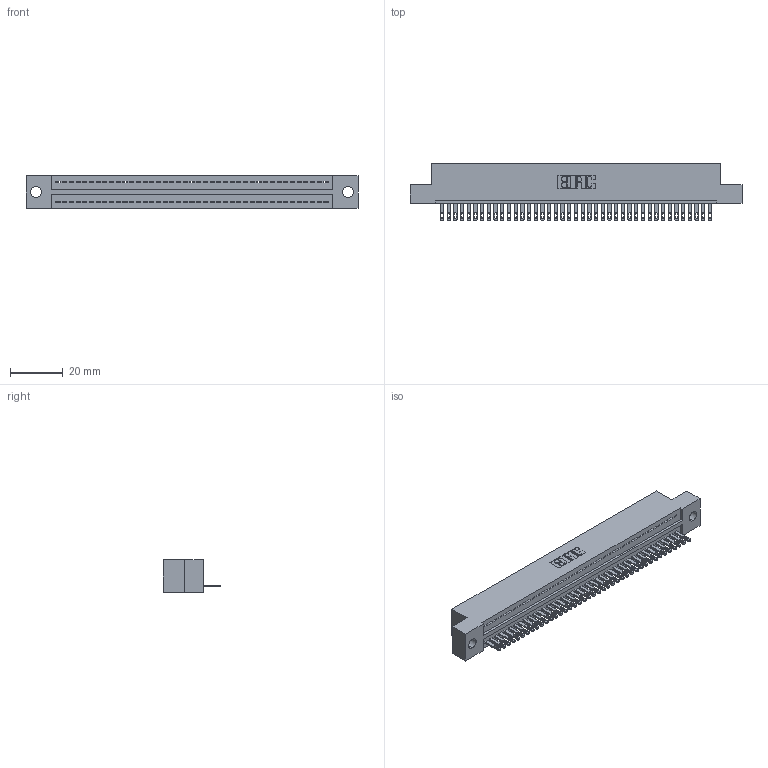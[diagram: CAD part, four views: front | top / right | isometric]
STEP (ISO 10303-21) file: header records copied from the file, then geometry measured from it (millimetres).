
FILE_DESCRIPTION (( 'STEP AP203' ), '1' );
FILE_NAME ('325-041-500-109.STEP', '2020-02-24T21:39:10', ( '' ), ( '' ), 'SwSTEP 2.0', 'SolidWorks 2016', '' );
FILE_SCHEMA (( 'CONFIG_CONTROL_DESIGN' ));
Length unit declared in the file: inch
Products named in the file (3): 325 Part_.160 TH; 325-041-500-109; 325-292-001_325-293-100
Assembly tree (42 placements, depth 2):
  325-041-500-109
    325 Part_.160 TH
    325-292-001_325-293-100  x41
Bounding box: 125.86 x 21.84 x 12.45 mm (x, y, z)
Volume: 15764.4 mm3; surface area: 17197.3 mm2
Topology: 42 solids, 42 shells, 2328 faces, 7199 edges, 4798 vertices
Faces by surface type: plane 1546, cylinder 782
Entity records: 25127 total; most frequent: CARTESIAN_POINT 4341, ORIENTED_EDGE 4318, DIRECTION 3665, EDGE_CURVE 2159, LINE 2027, VECTOR 2027, VERTEX_POINT 1438, AXIS2_PLACEMENT_3D 819
